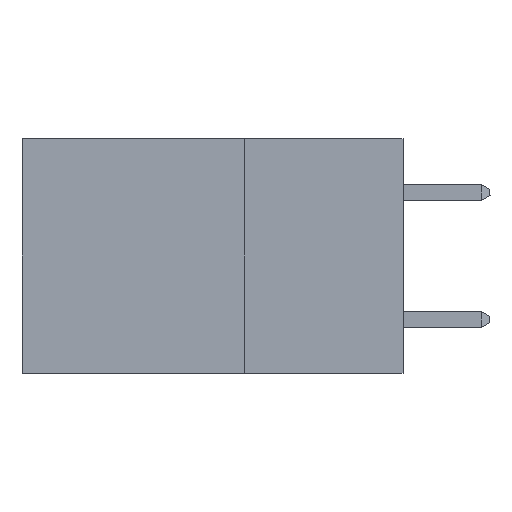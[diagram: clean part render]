
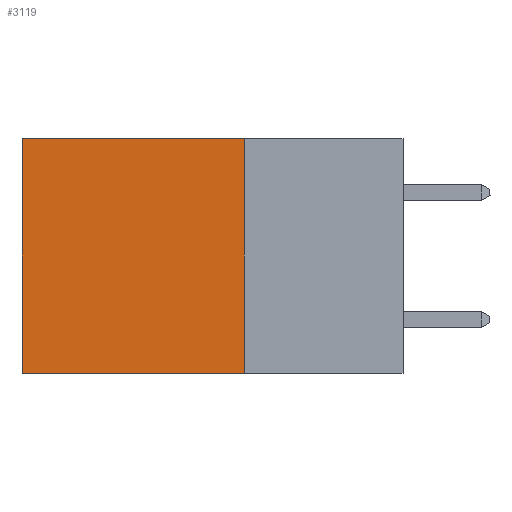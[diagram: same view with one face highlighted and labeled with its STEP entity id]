
A CAD part, left-side view. The second image highlights one B-rep face of the part: STEP entity #3119.
In plain terms, the highlighted planar face has unit normal (-1, 0, 0).
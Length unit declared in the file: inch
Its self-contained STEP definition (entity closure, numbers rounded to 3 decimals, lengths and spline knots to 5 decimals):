
#170 = DIRECTION ( 'NONE',  ( 1., 0., 0. ) ) ;
#258 = EDGE_CURVE ( 'NONE', #3019, #12965, #16186, .T. ) ;
#266 = DIRECTION ( 'NONE',  ( 0., 0., -1. ) ) ;
#1006 = CARTESIAN_POINT ( 'NONE',  ( 0.2875, 0.6, 0. ) ) ;
#1224 = DIRECTION ( 'NONE',  ( 0., 1., 0. ) ) ;
#2595 = CARTESIAN_POINT ( 'NONE',  ( 0.2875, 0.25, -0.37 ) ) ;
#2933 = ORIENTED_EDGE ( 'NONE', *, *, #10181, .T. ) ;
#3019 = VERTEX_POINT ( 'NONE', #11473 ) ;
#3119 = ADVANCED_FACE ( 'NONE', ( #11879 ), #14385, .F. ) ;
#3455 = VECTOR ( 'NONE', #9133, 39.37008 ) ;
#3864 = LINE ( 'NONE', #2595, #3455 ) ;
#4678 = CARTESIAN_POINT ( 'NONE',  ( 0.2875, 0.25, 0. ) ) ;
#5065 = EDGE_CURVE ( 'NONE', #11895, #12578, #11193, .T. ) ;
#5323 = VECTOR ( 'NONE', #9773, 39.37008 ) ;
#6607 = ORIENTED_EDGE ( 'NONE', *, *, #258, .F. ) ;
#8296 = ORIENTED_EDGE ( 'NONE', *, *, #5065, .T. ) ;
#9133 = DIRECTION ( 'NONE',  ( 0., 1., 0. ) ) ;
#9773 = DIRECTION ( 'NONE',  ( 0., 0., -1. ) ) ;
#10081 = LINE ( 'NONE', #11410, #10658 ) ;
#10142 = CARTESIAN_POINT ( 'NONE',  ( 0.2875, 0.6, -0.37 ) ) ;
#10181 = EDGE_CURVE ( 'NONE', #3019, #11895, #10081, .T. ) ;
#10658 = VECTOR ( 'NONE', #1224, 39.37008 ) ;
#11051 = ORIENTED_EDGE ( 'NONE', *, *, #14966, .F. ) ;
#11193 = LINE ( 'NONE', #1006, #14252 ) ;
#11410 = CARTESIAN_POINT ( 'NONE',  ( 0.2875, 0.25, 0. ) ) ;
#11473 = CARTESIAN_POINT ( 'NONE',  ( 0.2875, 0.25, 0. ) ) ;
#11879 = FACE_OUTER_BOUND ( 'NONE', #15193, .T. ) ;
#11895 = VERTEX_POINT ( 'NONE', #16094 ) ;
#12527 = DIRECTION ( 'NONE',  ( 0., 0., -1. ) ) ;
#12578 = VERTEX_POINT ( 'NONE', #10142 ) ;
#12965 = VERTEX_POINT ( 'NONE', #14334 ) ;
#14252 = VECTOR ( 'NONE', #12527, 39.37008 ) ;
#14334 = CARTESIAN_POINT ( 'NONE',  ( 0.2875, 0.25, -0.37 ) ) ;
#14385 = PLANE ( 'NONE',  #14456 ) ;
#14456 = AXIS2_PLACEMENT_3D ( 'NONE', #15554, #170, #266 ) ;
#14966 = EDGE_CURVE ( 'NONE', #12965, #12578, #3864, .T. ) ;
#15193 = EDGE_LOOP ( 'NONE', ( #8296, #11051, #6607, #2933 ) ) ;
#15554 = CARTESIAN_POINT ( 'NONE',  ( 0.2875, 0.25, 0. ) ) ;
#16094 = CARTESIAN_POINT ( 'NONE',  ( 0.2875, 0.6, 0. ) ) ;
#16186 = LINE ( 'NONE', #4678, #5323 ) ;
